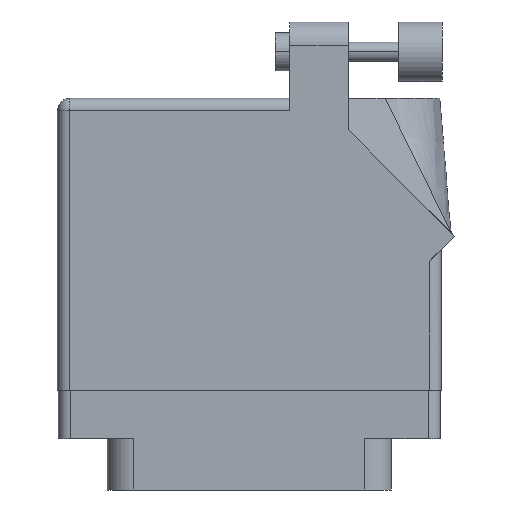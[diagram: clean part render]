
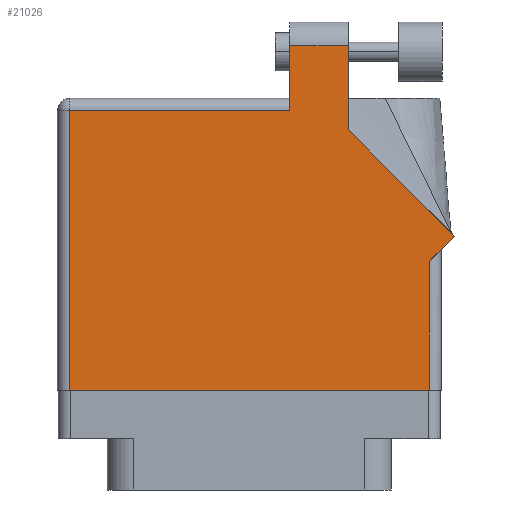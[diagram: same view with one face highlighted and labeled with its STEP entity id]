
A CAD part, front view. The second image highlights one B-rep face of the part: STEP entity #21026.
In plain terms, the highlighted face is planar.
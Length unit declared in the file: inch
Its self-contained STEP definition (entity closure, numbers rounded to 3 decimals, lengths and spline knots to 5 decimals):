
#313 = CARTESIAN_POINT ( 'NONE',  ( -1.005, 1.43, 0.455 ) ) ;
#442 = ORIENTED_EDGE ( 'NONE', *, *, #21320, .T. ) ;
#638 = DIRECTION ( 'NONE',  ( -1., 0., 0. ) ) ;
#1518 = LINE ( 'NONE', #8424, #20529 ) ;
#1913 = ORIENTED_EDGE ( 'NONE', *, *, #17126, .T. ) ;
#2303 = CARTESIAN_POINT ( 'NONE',  ( 1.07571, 0.70771, 0.455 ) ) ;
#2733 = CARTESIAN_POINT ( 'NONE',  ( 0.519, 1.26442, 0.455 ) ) ;
#3328 = VERTEX_POINT ( 'NONE', #6170 ) ;
#4060 = CARTESIAN_POINT ( 'NONE',  ( 0.519, 1.705, 0.455 ) ) ;
#4348 = LINE ( 'NONE', #31660, #10536 ) ;
#5280 = VECTOR ( 'NONE', #11523, 39.37008 ) ;
#5964 = VECTOR ( 'NONE', #27279, 39.37008 ) ;
#6170 = CARTESIAN_POINT ( 'NONE',  ( -0.943, 1.368, 0.455 ) ) ;
#6245 = CARTESIAN_POINT ( 'NONE',  ( 1.07571, 0.70771, 0.455 ) ) ;
#6840 = CARTESIAN_POINT ( 'NONE',  ( 0.212, 1.705, 0.455 ) ) ;
#7611 = CARTESIAN_POINT ( 'NONE',  ( 0.943, -0.1, 0.455 ) ) ;
#8424 = CARTESIAN_POINT ( 'NONE',  ( -1.005, 1.368, 0.455 ) ) ;
#8613 = LINE ( 'NONE', #19443, #31139 ) ;
#8753 = DIRECTION ( 'NONE',  ( -1., 0., 0. ) ) ;
#8963 = ORIENTED_EDGE ( 'NONE', *, *, #13619, .T. ) ;
#9006 = CARTESIAN_POINT ( 'NONE',  ( -0.943, -0.1, 0.455 ) ) ;
#9080 = DIRECTION ( 'NONE',  ( 1., 0., 0. ) ) ;
#9227 = CARTESIAN_POINT ( 'NONE',  ( 0.943, 0.637, 0.455 ) ) ;
#9278 = CARTESIAN_POINT ( 'NONE',  ( 1.005, 0.637, 0.455 ) ) ;
#10186 = ORIENTED_EDGE ( 'NONE', *, *, #15210, .T. ) ;
#10536 = VECTOR ( 'NONE', #9080, 39.37008 ) ;
#11523 = DIRECTION ( 'NONE',  ( 0., -1., 0. ) ) ;
#11549 = LINE ( 'NONE', #28399, #28219 ) ;
#11763 = VERTEX_POINT ( 'NONE', #9006 ) ;
#11815 = VERTEX_POINT ( 'NONE', #6840 ) ;
#11839 = CARTESIAN_POINT ( 'NONE',  ( 0.212, 1.43, 0.455 ) ) ;
#12789 = DIRECTION ( 'NONE',  ( 0., 0., -1. ) ) ;
#13119 = DIRECTION ( 'NONE',  ( 0., -1., 0. ) ) ;
#13198 = EDGE_CURVE ( 'NONE', #11763, #16736, #4348, .T. ) ;
#13619 = EDGE_CURVE ( 'NONE', #14446, #15639, #18301, .T. ) ;
#13754 = DIRECTION ( 'NONE',  ( -0.707, 0.707, 0. ) ) ;
#14446 = VERTEX_POINT ( 'NONE', #2303 ) ;
#15006 = ORIENTED_EDGE ( 'NONE', *, *, #13198, .T. ) ;
#15210 = EDGE_CURVE ( 'NONE', #20997, #3328, #1518, .T. ) ;
#15639 = VERTEX_POINT ( 'NONE', #2733 ) ;
#15747 = ORIENTED_EDGE ( 'NONE', *, *, #30730, .T. ) ;
#16026 = DIRECTION ( 'NONE',  ( -1., 0., 0. ) ) ;
#16475 = VERTEX_POINT ( 'NONE', #4060 ) ;
#16577 = CARTESIAN_POINT ( 'NONE',  ( 0.212, 1.705, 0.455 ) ) ;
#16614 = AXIS2_PLACEMENT_3D ( 'NONE', #313, #12789, #638 ) ;
#16736 = VERTEX_POINT ( 'NONE', #7611 ) ;
#16798 = LINE ( 'NONE', #9227, #19904 ) ;
#17126 = EDGE_CURVE ( 'NONE', #11815, #20997, #29362, .T. ) ;
#17578 = PLANE ( 'NONE',  #16614 ) ;
#17843 = LINE ( 'NONE', #16577, #30229 ) ;
#18279 = VERTEX_POINT ( 'NONE', #18971 ) ;
#18288 = EDGE_CURVE ( 'NONE', #18279, #14446, #22668, .T. ) ;
#18301 = LINE ( 'NONE', #6245, #22921 ) ;
#18971 = CARTESIAN_POINT ( 'NONE',  ( 0.943, 0.575, 0.455 ) ) ;
#19095 = ORIENTED_EDGE ( 'NONE', *, *, #19210, .T. ) ;
#19210 = EDGE_CURVE ( 'NONE', #16736, #18279, #16798, .T. ) ;
#19232 = DIRECTION ( 'NONE',  ( 0., 1., 0. ) ) ;
#19322 = EDGE_CURVE ( 'NONE', #15639, #16475, #8613, .T. ) ;
#19443 = CARTESIAN_POINT ( 'NONE',  ( 0.519, 1.26442, 0.455 ) ) ;
#19904 = VECTOR ( 'NONE', #19232, 39.37008 ) ;
#19970 = ORIENTED_EDGE ( 'NONE', *, *, #19322, .T. ) ;
#20529 = VECTOR ( 'NONE', #16026, 39.37008 ) ;
#20997 = VERTEX_POINT ( 'NONE', #24826 ) ;
#21026 = ADVANCED_FACE ( 'NONE', ( #25601 ), #17578, .F. ) ;
#21320 = EDGE_CURVE ( 'NONE', #16475, #11815, #17843, .T. ) ;
#21612 = DIRECTION ( 'NONE',  ( 0., 1., 0. ) ) ;
#22668 = LINE ( 'NONE', #9278, #5964 ) ;
#22921 = VECTOR ( 'NONE', #13754, 39.37008 ) ;
#24436 = EDGE_LOOP ( 'NONE', ( #19970, #442, #1913, #10186, #15747, #15006, #19095, #25326, #8963 ) ) ;
#24826 = CARTESIAN_POINT ( 'NONE',  ( 0.212, 1.368, 0.455 ) ) ;
#25326 = ORIENTED_EDGE ( 'NONE', *, *, #18288, .T. ) ;
#25601 = FACE_OUTER_BOUND ( 'NONE', #24436, .T. ) ;
#27279 = DIRECTION ( 'NONE',  ( 0.707, 0.707, 0. ) ) ;
#28219 = VECTOR ( 'NONE', #13119, 39.37008 ) ;
#28399 = CARTESIAN_POINT ( 'NONE',  ( -0.943, -0.1, 0.455 ) ) ;
#29362 = LINE ( 'NONE', #11839, #5280 ) ;
#30229 = VECTOR ( 'NONE', #8753, 39.37008 ) ;
#30730 = EDGE_CURVE ( 'NONE', #3328, #11763, #11549, .T. ) ;
#31139 = VECTOR ( 'NONE', #21612, 39.37008 ) ;
#31660 = CARTESIAN_POINT ( 'NONE',  ( -1.005, -0.1, 0.455 ) ) ;
